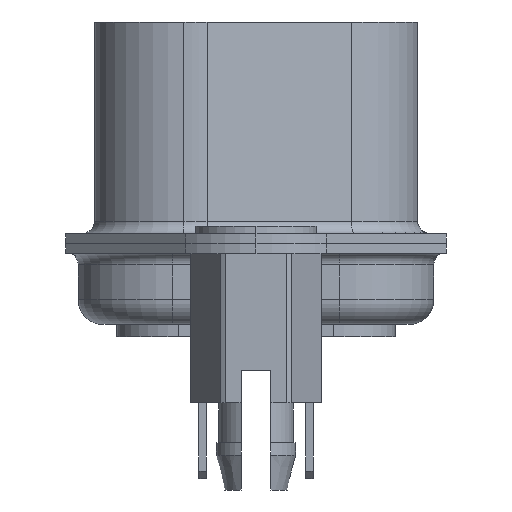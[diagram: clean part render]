
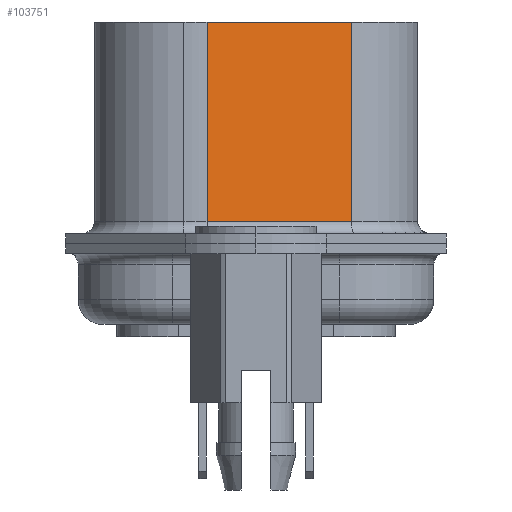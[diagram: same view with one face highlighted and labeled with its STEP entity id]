
A CAD part, left-side view. The second image highlights one B-rep face of the part: STEP entity #103751.
In plain terms, the highlighted planar face has unit normal (-0.966, -0.259, 0).
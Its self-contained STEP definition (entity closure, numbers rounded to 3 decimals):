
#10573 = CARTESIAN_POINT ( 'NONE',  ( 6.467, -3.832, 9.3 ) ) ;
#25760 = FACE_OUTER_BOUND ( 'NONE', #31586, .T. ) ;
#31586 = EDGE_LOOP ( 'NONE', ( #82722, #146116, #120109, #41867 ) ) ;
#39497 = DIRECTION ( 'NONE',  ( 0., 0., -1. ) ) ;
#40480 = DIRECTION ( 'NONE',  ( 0., 0., -1. ) ) ;
#41867 = ORIENTED_EDGE ( 'NONE', *, *, #126588, .F. ) ;
#46469 = CARTESIAN_POINT ( 'NONE',  ( 6.467, -3.832, 9.3 ) ) ;
#48236 = PLANE ( 'NONE',  #61800 ) ;
#49813 = DIRECTION ( 'NONE',  ( -0.259, 0.966, 0. ) ) ;
#54698 = CARTESIAN_POINT ( 'NONE',  ( 4.913, 1.968, 9.3 ) ) ;
#61800 = AXIS2_PLACEMENT_3D ( 'NONE', #10573, #98692, #49813 ) ;
#67721 = EDGE_CURVE ( 'NONE', #149812, #127230, #141085, .T. ) ;
#68787 = VERTEX_POINT ( 'NONE', #142437 ) ;
#77343 = LINE ( 'NONE', #103753, #133465 ) ;
#77634 = CARTESIAN_POINT ( 'NONE',  ( 4.913, 1.968, 9.3 ) ) ;
#80930 = VERTEX_POINT ( 'NONE', #77634 ) ;
#82722 = ORIENTED_EDGE ( 'NONE', *, *, #86667, .T. ) ;
#86667 = EDGE_CURVE ( 'NONE', #80930, #149812, #151631, .T. ) ;
#93048 = CARTESIAN_POINT ( 'NONE',  ( 6.467, -3.832, 1.3 ) ) ;
#95374 = VECTOR ( 'NONE', #120944, 1000. ) ;
#95513 = CARTESIAN_POINT ( 'NONE',  ( 4.913, 1.968, 1.3 ) ) ;
#98692 = DIRECTION ( 'NONE',  ( 0.966, 0.259, 0. ) ) ;
#103631 = CARTESIAN_POINT ( 'NONE',  ( 6.467, -3.832, 1.3 ) ) ;
#103751 = ADVANCED_FACE ( 'NONE', ( #25760 ), #48236, .F. ) ;
#103753 = CARTESIAN_POINT ( 'NONE',  ( 6.467, -3.832, 9.3 ) ) ;
#111482 = VECTOR ( 'NONE', #39497, 1000. ) ;
#118589 = LINE ( 'NONE', #46469, #95374 ) ;
#120109 = ORIENTED_EDGE ( 'NONE', *, *, #136260, .F. ) ;
#120944 = DIRECTION ( 'NONE',  ( 0.259, -0.966, 0. ) ) ;
#126588 = EDGE_CURVE ( 'NONE', #80930, #68787, #118589, .T. ) ;
#127230 = VERTEX_POINT ( 'NONE', #103631 ) ;
#129838 = DIRECTION ( 'NONE',  ( 0.259, -0.966, 0. ) ) ;
#133465 = VECTOR ( 'NONE', #40480, 1000. ) ;
#136260 = EDGE_CURVE ( 'NONE', #68787, #127230, #77343, .T. ) ;
#141085 = LINE ( 'NONE', #93048, #155738 ) ;
#142437 = CARTESIAN_POINT ( 'NONE',  ( 6.467, -3.832, 9.3 ) ) ;
#146116 = ORIENTED_EDGE ( 'NONE', *, *, #67721, .T. ) ;
#149812 = VERTEX_POINT ( 'NONE', #95513 ) ;
#151631 = LINE ( 'NONE', #54698, #111482 ) ;
#155738 = VECTOR ( 'NONE', #129838, 1000. ) ;
